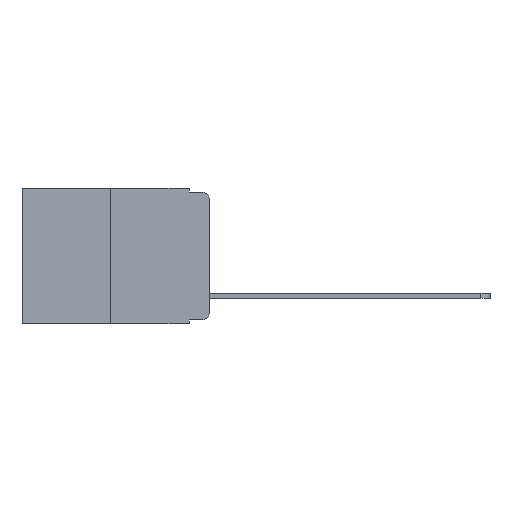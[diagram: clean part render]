
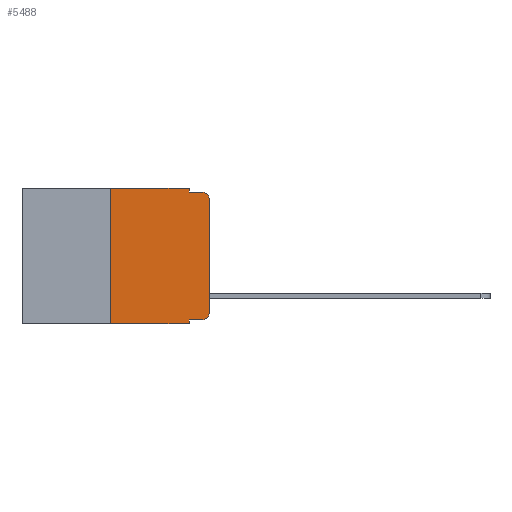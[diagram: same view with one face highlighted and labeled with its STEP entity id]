
A CAD part, left-side view. The second image highlights one B-rep face of the part: STEP entity #5488.
In plain terms, the highlighted planar face has unit normal (-1, 0, 0).
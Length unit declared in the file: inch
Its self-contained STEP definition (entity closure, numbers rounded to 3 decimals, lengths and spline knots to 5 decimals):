
#232 = VERTEX_POINT ( 'NONE', #2726 ) ;
#439 = VERTEX_POINT ( 'NONE', #2295 ) ;
#1021 = LINE ( 'NONE', #6310, #3480 ) ;
#1047 = DIRECTION ( 'NONE',  ( 0., 0., -1. ) ) ;
#1127 = VERTEX_POINT ( 'NONE', #2166 ) ;
#1570 = AXIS2_PLACEMENT_3D ( 'NONE', #4762, #9904, #5578 ) ;
#1571 = CARTESIAN_POINT ( 'NONE',  ( 0., 0.051, 0. ) ) ;
#1766 = FACE_OUTER_BOUND ( 'NONE', #3866, .T. ) ;
#1792 = VECTOR ( 'NONE', #8929, 39.37008 ) ;
#1829 = AXIS2_PLACEMENT_3D ( 'NONE', #9910, #5594, #10585 ) ;
#1995 = DIRECTION ( 'NONE',  ( 0., -1., 0. ) ) ;
#2166 = CARTESIAN_POINT ( 'NONE',  ( 0., 0.25, 0. ) ) ;
#2180 = DIRECTION ( 'NONE',  ( 0., 0., -1. ) ) ;
#2295 = CARTESIAN_POINT ( 'NONE',  ( 0., 0.051, -0.343 ) ) ;
#2302 = CARTESIAN_POINT ( 'NONE',  ( 0., 0.051, -0.333 ) ) ;
#2372 = VECTOR ( 'NONE', #8870, 39.37008 ) ;
#2529 = CARTESIAN_POINT ( 'NONE',  ( 0., 0.051, -0.01 ) ) ;
#2726 = CARTESIAN_POINT ( 'NONE',  ( 0., 0., -0.03 ) ) ;
#3213 = VECTOR ( 'NONE', #1995, 39.37008 ) ;
#3274 = LINE ( 'NONE', #7261, #5364 ) ;
#3472 = VERTEX_POINT ( 'NONE', #7929 ) ;
#3480 = VECTOR ( 'NONE', #1047, 39.37008 ) ;
#3520 = CARTESIAN_POINT ( 'NONE',  ( 0., 0., -0.313 ) ) ;
#3574 = ORIENTED_EDGE ( 'NONE', *, *, #8960, .T. ) ;
#3606 = ORIENTED_EDGE ( 'NONE', *, *, #8988, .T. ) ;
#3672 = ORIENTED_EDGE ( 'NONE', *, *, #9155, .F. ) ;
#3686 = ORIENTED_EDGE ( 'NONE', *, *, #9158, .F. ) ;
#3695 = ORIENTED_EDGE ( 'NONE', *, *, #7572, .F. ) ;
#3717 = ORIENTED_EDGE ( 'NONE', *, *, #9178, .F. ) ;
#3738 = ORIENTED_EDGE ( 'NONE', *, *, #8266, .T. ) ;
#3749 = ORIENTED_EDGE ( 'NONE', *, *, #9301, .F. ) ;
#3796 = ORIENTED_EDGE ( 'NONE', *, *, #9302, .T. ) ;
#3821 = ORIENTED_EDGE ( 'NONE', *, *, #9310, .T. ) ;
#3866 = EDGE_LOOP ( 'NONE', ( #3574, #3606, #3672, #3686, #3695, #3717, #3738, #3749, #3796, #3821 ) ) ;
#4139 = AXIS2_PLACEMENT_3D ( 'NONE', #4870, #4873, #2180 ) ;
#4216 = LINE ( 'NONE', #8897, #1792 ) ;
#4762 = CARTESIAN_POINT ( 'NONE',  ( 0., 0.02, -0.313 ) ) ;
#4798 = VECTOR ( 'NONE', #7437, 39.37008 ) ;
#4847 = VERTEX_POINT ( 'NONE', #2302 ) ;
#4870 = CARTESIAN_POINT ( 'NONE',  ( 0., 0.473, 0. ) ) ;
#4873 = DIRECTION ( 'NONE',  ( 1., 0., 0. ) ) ;
#4919 = VERTEX_POINT ( 'NONE', #5429 ) ;
#5097 = PLANE ( 'NONE',  #4139 ) ;
#5364 = VECTOR ( 'NONE', #7987, 39.37008 ) ;
#5429 = CARTESIAN_POINT ( 'NONE',  ( 0., 0.02, -0.01 ) ) ;
#5488 = ADVANCED_FACE ( 'NONE', ( #1766 ), #5097, .F. ) ;
#5522 = CARTESIAN_POINT ( 'NONE',  ( 0., 0., 0. ) ) ;
#5578 = DIRECTION ( 'NONE',  ( 0., 0., -1. ) ) ;
#5594 = DIRECTION ( 'NONE',  ( -1., 0., 0. ) ) ;
#5662 = VERTEX_POINT ( 'NONE', #8704 ) ;
#5673 = CIRCLE ( 'NONE', #1829, 0.02 ) ;
#6156 = VERTEX_POINT ( 'NONE', #2529 ) ;
#6170 = LINE ( 'NONE', #5522, #8349 ) ;
#6310 = CARTESIAN_POINT ( 'NONE',  ( 0., 0.051, 0. ) ) ;
#6339 = CARTESIAN_POINT ( 'NONE',  ( 0., 0.473, -0.343 ) ) ;
#6611 = CARTESIAN_POINT ( 'NONE',  ( 0., 0.02, -0.333 ) ) ;
#6629 = LINE ( 'NONE', #1571, #4798 ) ;
#6769 = VECTOR ( 'NONE', #7122, 39.37008 ) ;
#7122 = DIRECTION ( 'NONE',  ( 0., -1., 0. ) ) ;
#7196 = VERTEX_POINT ( 'NONE', #6611 ) ;
#7261 = CARTESIAN_POINT ( 'NONE',  ( 0., 0.473, 0. ) ) ;
#7437 = DIRECTION ( 'NONE',  ( 0., 0., -1. ) ) ;
#7521 = LINE ( 'NONE', #8484, #3213 ) ;
#7572 = EDGE_CURVE ( 'NONE', #1127, #3472, #3274, .T. ) ;
#7929 = CARTESIAN_POINT ( 'NONE',  ( 0., 0.051, 0. ) ) ;
#7987 = DIRECTION ( 'NONE',  ( 0., -1., 0. ) ) ;
#8143 = CARTESIAN_POINT ( 'NONE',  ( 0., 0.051, -0.01 ) ) ;
#8266 = EDGE_CURVE ( 'NONE', #5662, #439, #8918, .T. ) ;
#8349 = VECTOR ( 'NONE', #10512, 39.37008 ) ;
#8484 = CARTESIAN_POINT ( 'NONE',  ( 0., 0.051, -0.333 ) ) ;
#8704 = CARTESIAN_POINT ( 'NONE',  ( 0., 0.25, -0.343 ) ) ;
#8797 = LINE ( 'NONE', #8143, #2372 ) ;
#8865 = VERTEX_POINT ( 'NONE', #3520 ) ;
#8870 = DIRECTION ( 'NONE',  ( 0., -1., 0. ) ) ;
#8897 = CARTESIAN_POINT ( 'NONE',  ( 0., 0.25, 0. ) ) ;
#8918 = LINE ( 'NONE', #6339, #6769 ) ;
#8929 = DIRECTION ( 'NONE',  ( 0., 0., 1. ) ) ;
#8960 = EDGE_CURVE ( 'NONE', #8865, #232, #6170, .T. ) ;
#8988 = EDGE_CURVE ( 'NONE', #232, #4919, #5673, .T. ) ;
#9155 = EDGE_CURVE ( 'NONE', #6156, #4919, #8797, .T. ) ;
#9158 = EDGE_CURVE ( 'NONE', #3472, #6156, #6629, .T. ) ;
#9178 = EDGE_CURVE ( 'NONE', #5662, #1127, #4216, .T. ) ;
#9223 = CIRCLE ( 'NONE', #1570, 0.02 ) ;
#9301 = EDGE_CURVE ( 'NONE', #4847, #439, #1021, .T. ) ;
#9302 = EDGE_CURVE ( 'NONE', #4847, #7196, #7521, .T. ) ;
#9310 = EDGE_CURVE ( 'NONE', #7196, #8865, #9223, .T. ) ;
#9904 = DIRECTION ( 'NONE',  ( -1., 0., 0. ) ) ;
#9910 = CARTESIAN_POINT ( 'NONE',  ( 0., 0.02, -0.03 ) ) ;
#10512 = DIRECTION ( 'NONE',  ( 0., 0., 1. ) ) ;
#10585 = DIRECTION ( 'NONE',  ( 0., 0., -1. ) ) ;
